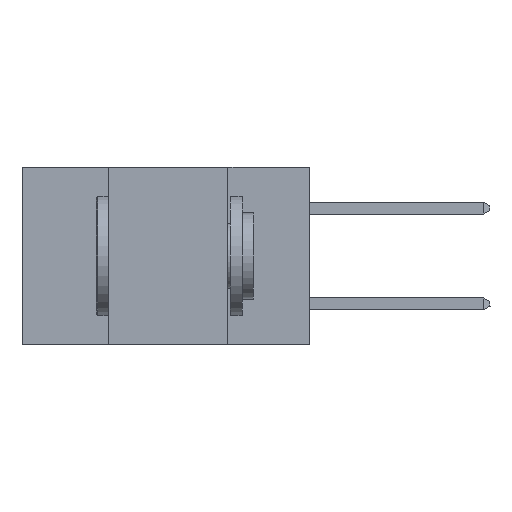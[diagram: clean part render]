
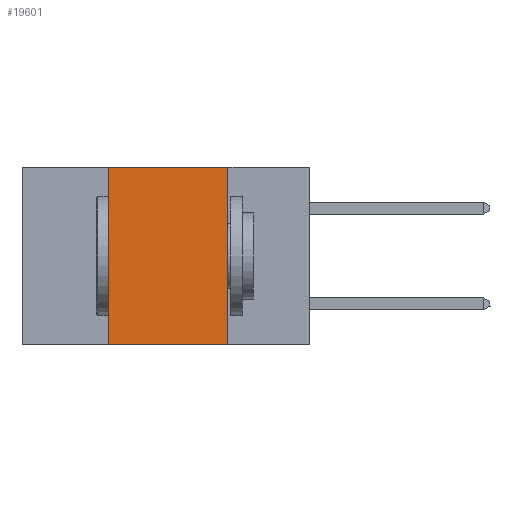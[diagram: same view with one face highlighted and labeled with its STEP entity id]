
A CAD part, left-side view. The second image highlights one B-rep face of the part: STEP entity #19601.
In plain terms, the highlighted planar face has unit normal (-1, 0, 0).
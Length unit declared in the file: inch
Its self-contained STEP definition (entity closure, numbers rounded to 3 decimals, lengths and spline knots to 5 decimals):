
#1391 = CARTESIAN_POINT ( 'NONE',  ( 0., 0.6, -0.37 ) ) ;
#2300 = AXIS2_PLACEMENT_3D ( 'NONE', #11368, #11451, #18752 ) ;
#2854 = EDGE_LOOP ( 'NONE', ( #22612, #12882, #7564, #4706 ) ) ;
#4094 = VERTEX_POINT ( 'NONE', #14467 ) ;
#4114 = LINE ( 'NONE', #1391, #5509 ) ;
#4555 = CARTESIAN_POINT ( 'NONE',  ( 0., 0.17, 0. ) ) ;
#4706 = ORIENTED_EDGE ( 'NONE', *, *, #12986, .T. ) ;
#5066 = CARTESIAN_POINT ( 'NONE',  ( 0., 0.42, 0. ) ) ;
#5509 = VECTOR ( 'NONE', #21263, 39.37008 ) ;
#5822 = EDGE_CURVE ( 'NONE', #16812, #15536, #11674, .T. ) ;
#5860 = DIRECTION ( 'NONE',  ( 0., -1., 0. ) ) ;
#6033 = CARTESIAN_POINT ( 'NONE',  ( 0., 0.42, 0. ) ) ;
#7238 = EDGE_CURVE ( 'NONE', #10065, #4094, #17868, .T. ) ;
#7564 = ORIENTED_EDGE ( 'NONE', *, *, #5822, .F. ) ;
#7965 = CARTESIAN_POINT ( 'NONE',  ( 0., 0.42, -0.37 ) ) ;
#8236 = EDGE_CURVE ( 'NONE', #15536, #10065, #9392, .T. ) ;
#8999 = CARTESIAN_POINT ( 'NONE',  ( 0., 0.17, 0. ) ) ;
#9392 = LINE ( 'NONE', #10850, #9673 ) ;
#9673 = VECTOR ( 'NONE', #5860, 39.37008 ) ;
#10065 = VERTEX_POINT ( 'NONE', #8999 ) ;
#10850 = CARTESIAN_POINT ( 'NONE',  ( 0., 0.6, 0. ) ) ;
#11368 = CARTESIAN_POINT ( 'NONE',  ( 0., 0.6, 0. ) ) ;
#11451 = DIRECTION ( 'NONE',  ( 1., 0., 0. ) ) ;
#11674 = LINE ( 'NONE', #6033, #20701 ) ;
#12882 = ORIENTED_EDGE ( 'NONE', *, *, #8236, .F. ) ;
#12986 = EDGE_CURVE ( 'NONE', #16812, #4094, #4114, .T. ) ;
#14159 = VECTOR ( 'NONE', #21183, 39.37008 ) ;
#14467 = CARTESIAN_POINT ( 'NONE',  ( 0., 0.17, -0.37 ) ) ;
#15536 = VERTEX_POINT ( 'NONE', #5066 ) ;
#16812 = VERTEX_POINT ( 'NONE', #7965 ) ;
#16838 = PLANE ( 'NONE',  #2300 ) ;
#17868 = LINE ( 'NONE', #4555, #14159 ) ;
#18752 = DIRECTION ( 'NONE',  ( 0., 0., -1. ) ) ;
#19027 = FACE_OUTER_BOUND ( 'NONE', #2854, .T. ) ;
#19601 = ADVANCED_FACE ( 'NONE', ( #19027 ), #16838, .F. ) ;
#20701 = VECTOR ( 'NONE', #22177, 39.37008 ) ;
#21183 = DIRECTION ( 'NONE',  ( 0., 0., -1. ) ) ;
#21263 = DIRECTION ( 'NONE',  ( 0., -1., 0. ) ) ;
#22177 = DIRECTION ( 'NONE',  ( 0., 0., 1. ) ) ;
#22612 = ORIENTED_EDGE ( 'NONE', *, *, #7238, .F. ) ;
